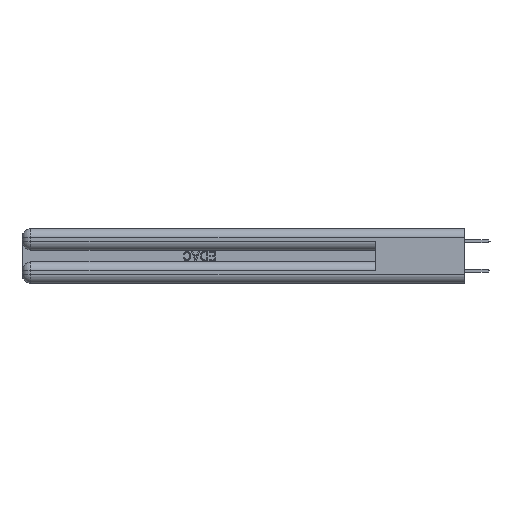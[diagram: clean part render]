
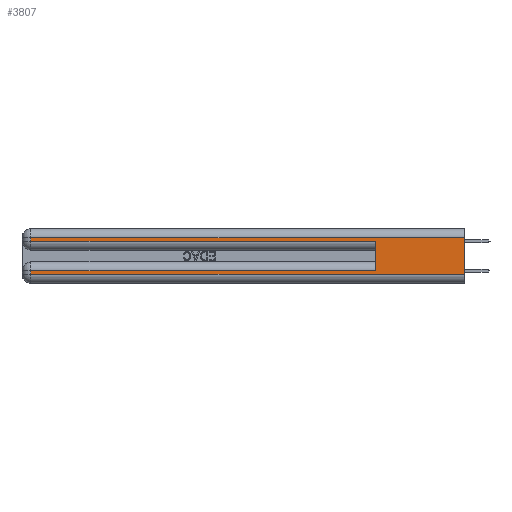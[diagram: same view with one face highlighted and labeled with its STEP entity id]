
A CAD part, left-side view. The second image highlights one B-rep face of the part: STEP entity #3807.
In plain terms, the highlighted planar face has unit normal (-1, 0, 0).
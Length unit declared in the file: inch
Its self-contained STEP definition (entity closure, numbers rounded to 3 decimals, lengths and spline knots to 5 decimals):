
#2815 = DIRECTION ( 'NONE',  ( 0., 0., -1. ) ) ;
#3807 = ADVANCED_FACE ( 'NONE', ( #19543 ), #43576, .F. ) ;
#4322 = VERTEX_POINT ( 'NONE', #36246 ) ;
#4396 = DIRECTION ( 'NONE',  ( 0., 1., 0. ) ) ;
#4641 = DIRECTION ( 'NONE',  ( 0., 1., 0. ) ) ;
#5010 = CARTESIAN_POINT ( 'NONE',  ( 0., 2.94, 0.285 ) ) ;
#5923 = EDGE_CURVE ( 'NONE', #4322, #43267, #14623, .T. ) ;
#6344 = VECTOR ( 'NONE', #4641, 39.37008 ) ;
#6412 = ORIENTED_EDGE ( 'NONE', *, *, #25549, .F. ) ;
#6641 = EDGE_CURVE ( 'NONE', #35593, #27740, #19890, .T. ) ;
#7067 = ORIENTED_EDGE ( 'NONE', *, *, #6641, .T. ) ;
#7826 = CARTESIAN_POINT ( 'NONE',  ( 0., 0., 0.285 ) ) ;
#9329 = EDGE_CURVE ( 'NONE', #28832, #29522, #12026, .T. ) ;
#9825 = ORIENTED_EDGE ( 'NONE', *, *, #9329, .T. ) ;
#10055 = CARTESIAN_POINT ( 'NONE',  ( 0., 2.94, 0.37 ) ) ;
#11738 = ORIENTED_EDGE ( 'NONE', *, *, #37179, .T. ) ;
#12026 = LINE ( 'NONE', #7826, #37019 ) ;
#12785 = CARTESIAN_POINT ( 'NONE',  ( 0., 0., 0.06 ) ) ;
#13225 = DIRECTION ( 'NONE',  ( 0., 0., 1. ) ) ;
#14623 = LINE ( 'NONE', #38376, #18362 ) ;
#15046 = CARTESIAN_POINT ( 'NONE',  ( 0., 0., 0.085 ) ) ;
#15742 = CARTESIAN_POINT ( 'NONE',  ( 0., 0., 0.37 ) ) ;
#16035 = ORIENTED_EDGE ( 'NONE', *, *, #28213, .F. ) ;
#16518 = CARTESIAN_POINT ( 'NONE',  ( 0., 0., 0.37 ) ) ;
#17915 = CARTESIAN_POINT ( 'NONE',  ( 0., 2.94, 0.085 ) ) ;
#18362 = VECTOR ( 'NONE', #4396, 39.37008 ) ;
#18435 = VECTOR ( 'NONE', #31871, 39.37008 ) ;
#19543 = FACE_OUTER_BOUND ( 'NONE', #32390, .T. ) ;
#19890 = LINE ( 'NONE', #12785, #37891 ) ;
#19900 = ORIENTED_EDGE ( 'NONE', *, *, #5923, .T. ) ;
#20319 = CARTESIAN_POINT ( 'NONE',  ( 0., 0.6, 0.085 ) ) ;
#20858 = CARTESIAN_POINT ( 'NONE',  ( 0., 2.94, 0.31 ) ) ;
#21632 = CARTESIAN_POINT ( 'NONE',  ( 0., 2.94, 0.37 ) ) ;
#23343 = DIRECTION ( 'NONE',  ( 1., 0., 0. ) ) ;
#24526 = LINE ( 'NONE', #15046, #6344 ) ;
#25549 = EDGE_CURVE ( 'NONE', #38745, #29522, #34607, .T. ) ;
#26439 = ORIENTED_EDGE ( 'NONE', *, *, #39741, .T. ) ;
#26624 = VECTOR ( 'NONE', #13225, 39.37008 ) ;
#27408 = LINE ( 'NONE', #21632, #18435 ) ;
#27740 = VERTEX_POINT ( 'NONE', #29908 ) ;
#28213 = EDGE_CURVE ( 'NONE', #4322, #27740, #34174, .T. ) ;
#28830 = ORIENTED_EDGE ( 'NONE', *, *, #29876, .T. ) ;
#28832 = VERTEX_POINT ( 'NONE', #5010 ) ;
#29522 = VERTEX_POINT ( 'NONE', #35522 ) ;
#29876 = EDGE_CURVE ( 'NONE', #43267, #28832, #44036, .T. ) ;
#29908 = CARTESIAN_POINT ( 'NONE',  ( 0., 0., 0.06 ) ) ;
#30519 = CARTESIAN_POINT ( 'NONE',  ( 0., 2.94, 0.06 ) ) ;
#31713 = AXIS2_PLACEMENT_3D ( 'NONE', #16518, #23343, #2815 ) ;
#31871 = DIRECTION ( 'NONE',  ( 0., 0., -1. ) ) ;
#32390 = EDGE_LOOP ( 'NONE', ( #16035, #19900, #28830, #9825, #6412, #26439, #11738, #7067 ) ) ;
#32699 = DIRECTION ( 'NONE',  ( 0., 0., -1. ) ) ;
#33349 = VERTEX_POINT ( 'NONE', #17915 ) ;
#33619 = CARTESIAN_POINT ( 'NONE',  ( 0., 0.6, 0.145 ) ) ;
#34090 = VECTOR ( 'NONE', #37251, 39.37008 ) ;
#34174 = LINE ( 'NONE', #15742, #42051 ) ;
#34607 = LINE ( 'NONE', #33619, #26624 ) ;
#35077 = DIRECTION ( 'NONE',  ( 0., -1., 0. ) ) ;
#35522 = CARTESIAN_POINT ( 'NONE',  ( 0., 0.6, 0.285 ) ) ;
#35593 = VERTEX_POINT ( 'NONE', #30519 ) ;
#36246 = CARTESIAN_POINT ( 'NONE',  ( 0., 0., 0.31 ) ) ;
#37019 = VECTOR ( 'NONE', #35077, 39.37008 ) ;
#37179 = EDGE_CURVE ( 'NONE', #33349, #35593, #27408, .T. ) ;
#37251 = DIRECTION ( 'NONE',  ( 0., 0., -1. ) ) ;
#37891 = VECTOR ( 'NONE', #39925, 39.37008 ) ;
#38376 = CARTESIAN_POINT ( 'NONE',  ( 0., 0., 0.31 ) ) ;
#38745 = VERTEX_POINT ( 'NONE', #20319 ) ;
#39741 = EDGE_CURVE ( 'NONE', #38745, #33349, #24526, .T. ) ;
#39925 = DIRECTION ( 'NONE',  ( 0., -1., 0. ) ) ;
#42051 = VECTOR ( 'NONE', #32699, 39.37008 ) ;
#43267 = VERTEX_POINT ( 'NONE', #20858 ) ;
#43576 = PLANE ( 'NONE',  #31713 ) ;
#44036 = LINE ( 'NONE', #10055, #34090 ) ;
